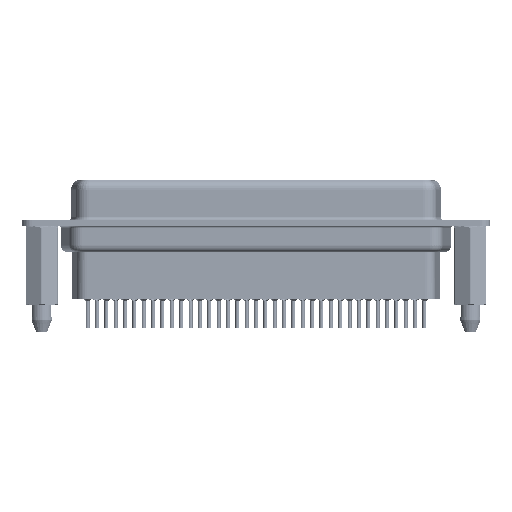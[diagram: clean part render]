
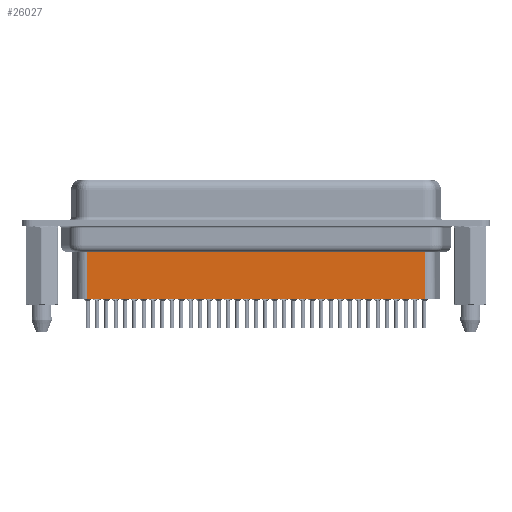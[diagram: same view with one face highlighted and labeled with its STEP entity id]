
A CAD part, front view. The second image highlights one B-rep face of the part: STEP entity #26027.
In plain terms, the highlighted planar face has unit normal (0, -1, 0).
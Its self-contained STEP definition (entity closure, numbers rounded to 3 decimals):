
#248 = DIRECTION ( 'NONE',  ( 0., 0., -1. ) ) ;
#639 = DIRECTION ( 'NONE',  ( 1., 0., 0. ) ) ;
#1800 = VECTOR ( 'NONE', #18975, 1000. ) ;
#2170 = EDGE_CURVE ( 'NONE', #28330, #4310, #3568, .T. ) ;
#3231 = CARTESIAN_POINT ( 'NONE',  ( 6.459, -3.5, -4.097 ) ) ;
#3568 = LINE ( 'NONE', #3231, #1800 ) ;
#3583 = ORIENTED_EDGE ( 'NONE', *, *, #12978, .F. ) ;
#4126 = CARTESIAN_POINT ( 'NONE',  ( 6.706, -3.5, -11.15 ) ) ;
#4289 = AXIS2_PLACEMENT_3D ( 'NONE', #21677, #28702, #639 ) ;
#4310 = VERTEX_POINT ( 'NONE', #31698 ) ;
#5344 = CARTESIAN_POINT ( 'NONE',  ( 6.706, -3.5, -3.1 ) ) ;
#6411 = ORIENTED_EDGE ( 'NONE', *, *, #20158, .F. ) ;
#7925 = LINE ( 'NONE', #5344, #13077 ) ;
#9592 = VERTEX_POINT ( 'NONE', #30242 ) ;
#12978 = EDGE_CURVE ( 'NONE', #28330, #18357, #13162, .T. ) ;
#13077 = VECTOR ( 'NONE', #248, 1000. ) ;
#13162 = LINE ( 'NONE', #13332, #32823 ) ;
#13332 = CARTESIAN_POINT ( 'NONE',  ( 56.794, -3.5, -3.1 ) ) ;
#15797 = ORIENTED_EDGE ( 'NONE', *, *, #17201, .T. ) ;
#16011 = PLANE ( 'NONE',  #4289 ) ;
#16355 = FACE_OUTER_BOUND ( 'NONE', #31426, .T. ) ;
#17201 = EDGE_CURVE ( 'NONE', #4310, #9592, #7925, .T. ) ;
#18357 = VERTEX_POINT ( 'NONE', #33688 ) ;
#18975 = DIRECTION ( 'NONE',  ( -1., 0., 0. ) ) ;
#20158 = EDGE_CURVE ( 'NONE', #18357, #9592, #29822, .T. ) ;
#20538 = CARTESIAN_POINT ( 'NONE',  ( 56.794, -3.5, -4.097 ) ) ;
#21677 = CARTESIAN_POINT ( 'NONE',  ( 6.706, -3.5, -3.1 ) ) ;
#26027 = ADVANCED_FACE ( 'NONE', ( #16355 ), #16011, .T. ) ;
#28330 = VERTEX_POINT ( 'NONE', #20538 ) ;
#28702 = DIRECTION ( 'NONE',  ( 0., -1., 0. ) ) ;
#29222 = ORIENTED_EDGE ( 'NONE', *, *, #2170, .T. ) ;
#29822 = LINE ( 'NONE', #4126, #30136 ) ;
#30136 = VECTOR ( 'NONE', #32930, 1000. ) ;
#30242 = CARTESIAN_POINT ( 'NONE',  ( 6.706, -3.5, -11.15 ) ) ;
#31426 = EDGE_LOOP ( 'NONE', ( #3583, #29222, #15797, #6411 ) ) ;
#31698 = CARTESIAN_POINT ( 'NONE',  ( 6.706, -3.5, -4.097 ) ) ;
#32823 = VECTOR ( 'NONE', #33594, 1000. ) ;
#32930 = DIRECTION ( 'NONE',  ( -1., 0., 0. ) ) ;
#33594 = DIRECTION ( 'NONE',  ( 0., 0., -1. ) ) ;
#33688 = CARTESIAN_POINT ( 'NONE',  ( 56.794, -3.5, -11.15 ) ) ;
